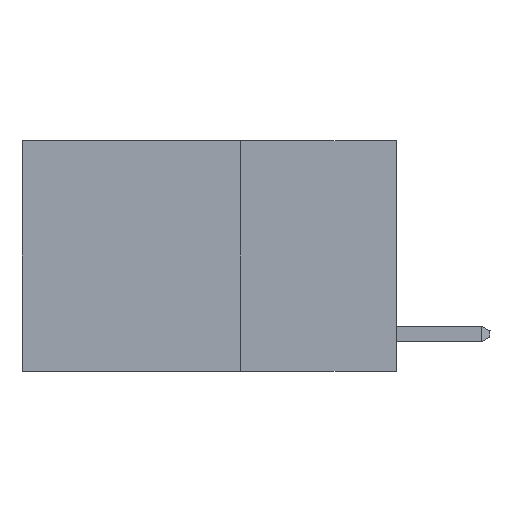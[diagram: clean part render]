
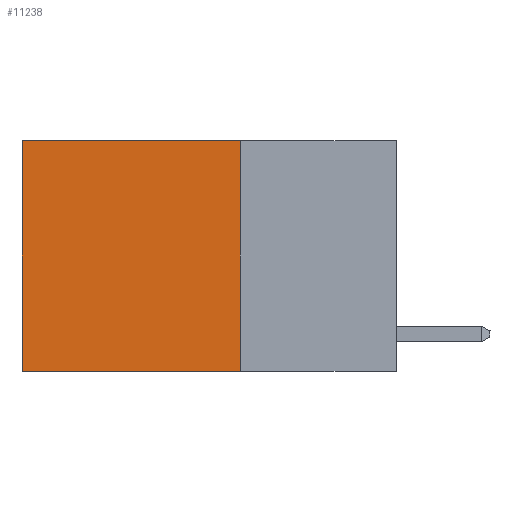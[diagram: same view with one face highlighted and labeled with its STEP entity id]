
A CAD part, left-side view. The second image highlights one B-rep face of the part: STEP entity #11238.
In plain terms, the highlighted planar face has unit normal (-1, 0, 0).
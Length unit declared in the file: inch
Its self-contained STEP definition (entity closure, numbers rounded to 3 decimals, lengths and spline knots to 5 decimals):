
#273 = EDGE_CURVE ( 'NONE', #3556, #14298, #13156, .T. ) ;
#447 = EDGE_LOOP ( 'NONE', ( #12872, #1229, #12940, #8872 ) ) ;
#1229 = ORIENTED_EDGE ( 'NONE', *, *, #3326, .F. ) ;
#2090 = CARTESIAN_POINT ( 'NONE',  ( 0.2625, 0.25, 0. ) ) ;
#2233 = DIRECTION ( 'NONE',  ( 0., 0., -1. ) ) ;
#2510 = AXIS2_PLACEMENT_3D ( 'NONE', #5669, #15834, #8329 ) ;
#3326 = EDGE_CURVE ( 'NONE', #5362, #8182, #12858, .T. ) ;
#3556 = VERTEX_POINT ( 'NONE', #2090 ) ;
#3926 = VECTOR ( 'NONE', #2233, 39.37008 ) ;
#4240 = DIRECTION ( 'NONE',  ( 0., 1., 0. ) ) ;
#4354 = LINE ( 'NONE', #13949, #9635 ) ;
#5062 = CARTESIAN_POINT ( 'NONE',  ( 0.2625, 0.25, -0.37 ) ) ;
#5362 = VERTEX_POINT ( 'NONE', #5062 ) ;
#5669 = CARTESIAN_POINT ( 'NONE',  ( 0.2625, 0.25, 0. ) ) ;
#6274 = CARTESIAN_POINT ( 'NONE',  ( 0.2625, 0.25, 0. ) ) ;
#7047 = PLANE ( 'NONE',  #2510 ) ;
#7620 = DIRECTION ( 'NONE',  ( 0., 1., 0. ) ) ;
#8063 = CARTESIAN_POINT ( 'NONE',  ( 0.2625, 0.25, -0.37 ) ) ;
#8182 = VERTEX_POINT ( 'NONE', #9932 ) ;
#8329 = DIRECTION ( 'NONE',  ( 0., 0., -1. ) ) ;
#8872 = ORIENTED_EDGE ( 'NONE', *, *, #273, .T. ) ;
#9505 = VECTOR ( 'NONE', #7620, 39.37008 ) ;
#9593 = VECTOR ( 'NONE', #4240, 39.37008 ) ;
#9635 = VECTOR ( 'NONE', #16462, 39.37008 ) ;
#9932 = CARTESIAN_POINT ( 'NONE',  ( 0.2625, 0.6, -0.37 ) ) ;
#9955 = CARTESIAN_POINT ( 'NONE',  ( 0.2625, 0.6, 0. ) ) ;
#11238 = ADVANCED_FACE ( 'NONE', ( #11282 ), #7047, .F. ) ;
#11282 = FACE_OUTER_BOUND ( 'NONE', #447, .T. ) ;
#12858 = LINE ( 'NONE', #8063, #9593 ) ;
#12872 = ORIENTED_EDGE ( 'NONE', *, *, #16193, .T. ) ;
#12940 = ORIENTED_EDGE ( 'NONE', *, *, #16267, .F. ) ;
#13156 = LINE ( 'NONE', #6274, #9505 ) ;
#13674 = LINE ( 'NONE', #13838, #3926 ) ;
#13838 = CARTESIAN_POINT ( 'NONE',  ( 0.2625, 0.6, 0. ) ) ;
#13949 = CARTESIAN_POINT ( 'NONE',  ( 0.2625, 0.25, 0. ) ) ;
#14298 = VERTEX_POINT ( 'NONE', #9955 ) ;
#15834 = DIRECTION ( 'NONE',  ( 1., 0., 0. ) ) ;
#16193 = EDGE_CURVE ( 'NONE', #14298, #8182, #13674, .T. ) ;
#16267 = EDGE_CURVE ( 'NONE', #3556, #5362, #4354, .T. ) ;
#16462 = DIRECTION ( 'NONE',  ( 0., 0., -1. ) ) ;
